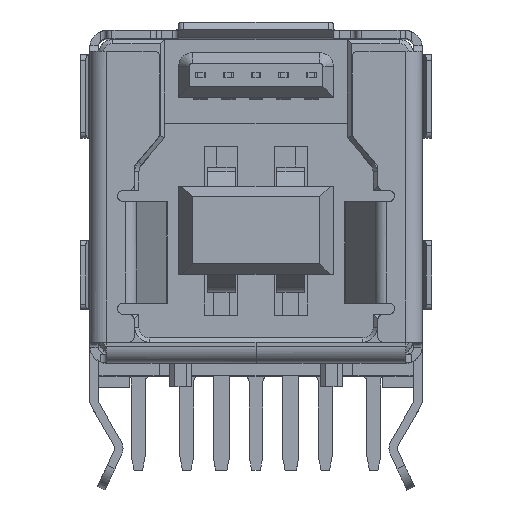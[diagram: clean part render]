
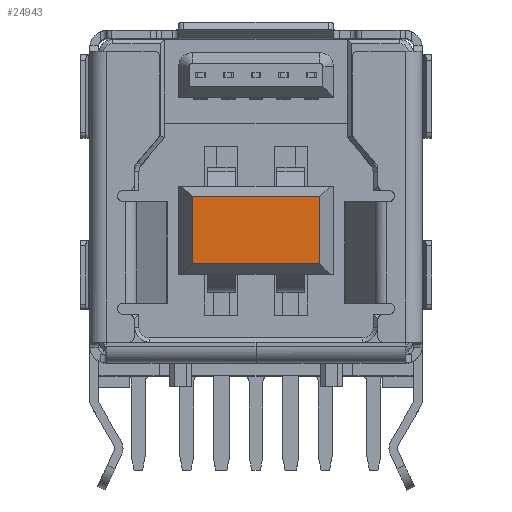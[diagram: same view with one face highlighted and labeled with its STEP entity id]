
A CAD part, top view. The second image highlights one B-rep face of the part: STEP entity #24943.
In plain terms, the highlighted planar face has unit normal (0, 0, 1).
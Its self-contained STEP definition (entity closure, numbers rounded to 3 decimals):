
#1528 = LINE ( 'NONE', #25904, #44207 ) ;
#1635 = VECTOR ( 'NONE', #43066, 1000. ) ;
#3117 = VERTEX_POINT ( 'NONE', #44321 ) ;
#5277 = ORIENTED_EDGE ( 'NONE', *, *, #35552, .T. ) ;
#7521 = CARTESIAN_POINT ( 'NONE',  ( -2.3, -2.42, -0.5 ) ) ;
#8368 = ORIENTED_EDGE ( 'NONE', *, *, #36137, .T. ) ;
#9844 = VECTOR ( 'NONE', #42920, 1000. ) ;
#12320 = VERTEX_POINT ( 'NONE', #41766 ) ;
#12668 = PLANE ( 'NONE',  #46017 ) ;
#12711 = CARTESIAN_POINT ( 'NONE',  ( 2.3, 0., -0.5 ) ) ;
#13268 = VERTEX_POINT ( 'NONE', #12711 ) ;
#17065 = ORIENTED_EDGE ( 'NONE', *, *, #23213, .T. ) ;
#18298 = EDGE_LOOP ( 'NONE', ( #8368, #33781, #5277, #17065 ) ) ;
#23213 = EDGE_CURVE ( 'NONE', #13268, #3117, #23233, .T. ) ;
#23233 = LINE ( 'NONE', #34008, #37780 ) ;
#24943 = ADVANCED_FACE ( 'NONE', ( #38231 ), #12668, .T. ) ;
#25904 = CARTESIAN_POINT ( 'NONE',  ( 2.3, -1.21, -0.5 ) ) ;
#26965 = CARTESIAN_POINT ( 'NONE',  ( -2.392, -2.468, -0.5 ) ) ;
#28761 = CARTESIAN_POINT ( 'NONE',  ( 0., -2.42, -0.5 ) ) ;
#28832 = VERTEX_POINT ( 'NONE', #7521 ) ;
#30478 = DIRECTION ( 'NONE',  ( 0., 0., 1. ) ) ;
#32378 = CARTESIAN_POINT ( 'NONE',  ( -2.3, -1.21, -0.5 ) ) ;
#33171 = DIRECTION ( 'NONE',  ( 0., 1., 0. ) ) ;
#33196 = LINE ( 'NONE', #28761, #1635 ) ;
#33781 = ORIENTED_EDGE ( 'NONE', *, *, #38038, .T. ) ;
#34008 = CARTESIAN_POINT ( 'NONE',  ( 0., 0., -0.5 ) ) ;
#35552 = EDGE_CURVE ( 'NONE', #12320, #13268, #1528, .T. ) ;
#36137 = EDGE_CURVE ( 'NONE', #3117, #28832, #45993, .T. ) ;
#37780 = VECTOR ( 'NONE', #44309, 1000. ) ;
#38038 = EDGE_CURVE ( 'NONE', #28832, #12320, #33196, .T. ) ;
#38231 = FACE_OUTER_BOUND ( 'NONE', #18298, .T. ) ;
#41766 = CARTESIAN_POINT ( 'NONE',  ( 2.3, -2.42, -0.5 ) ) ;
#42920 = DIRECTION ( 'NONE',  ( 0., -1., 0. ) ) ;
#43066 = DIRECTION ( 'NONE',  ( 1., 0., 0. ) ) ;
#44207 = VECTOR ( 'NONE', #33171, 1000. ) ;
#44309 = DIRECTION ( 'NONE',  ( -1., 0., 0. ) ) ;
#44321 = CARTESIAN_POINT ( 'NONE',  ( -2.3, 0., -0.5 ) ) ;
#44784 = DIRECTION ( 'NONE',  ( 1., 0., 0. ) ) ;
#45993 = LINE ( 'NONE', #32378, #9844 ) ;
#46017 = AXIS2_PLACEMENT_3D ( 'NONE', #26965, #30478, #44784 ) ;
